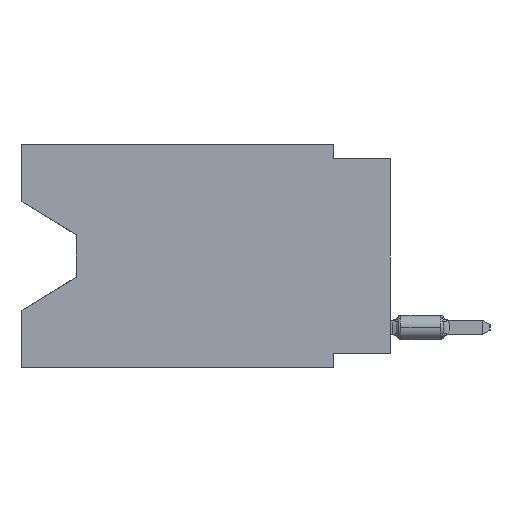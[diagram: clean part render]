
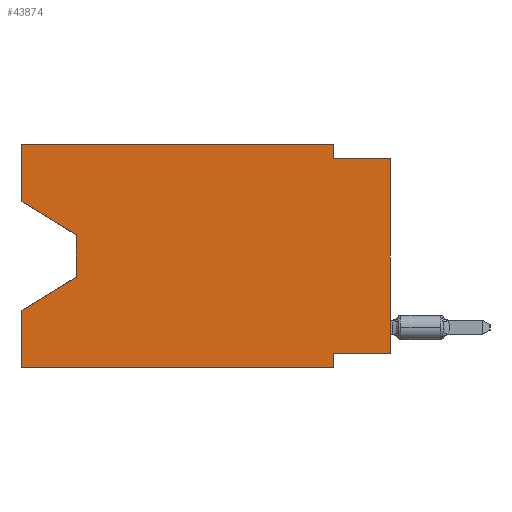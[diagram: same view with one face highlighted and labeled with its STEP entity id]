
A CAD part, left-side view. The second image highlights one B-rep face of the part: STEP entity #43874.
In plain terms, the highlighted planar face has unit normal (-1, 0, 0).
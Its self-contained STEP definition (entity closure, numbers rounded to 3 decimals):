
#273 = CARTESIAN_POINT ( 'NONE',  ( 0., 16.383, 0. ) ) ;
#1369 = LINE ( 'NONE', #19689, #4960 ) ;
#1424 = EDGE_LOOP ( 'NONE', ( #59179, #13717, #11758, #38852, #11616, #40115, #4180, #39235, #50964, #4521, #43627, #15643 ) ) ;
#2609 = CARTESIAN_POINT ( 'NONE',  ( 0., 16.383, -7.36 ) ) ;
#3058 = VERTEX_POINT ( 'NONE', #11367 ) ;
#3069 = CARTESIAN_POINT ( 'NONE',  ( 0., 16.383, 0. ) ) ;
#3442 = VECTOR ( 'NONE', #51423, 1000. ) ;
#4180 = ORIENTED_EDGE ( 'NONE', *, *, #4857, .F. ) ;
#4417 = DIRECTION ( 'NONE',  ( 0., 0., -1. ) ) ;
#4521 = ORIENTED_EDGE ( 'NONE', *, *, #47210, .F. ) ;
#4790 = EDGE_CURVE ( 'NONE', #7479, #24589, #44307, .T. ) ;
#4857 = EDGE_CURVE ( 'NONE', #54522, #42601, #21794, .T. ) ;
#4960 = VECTOR ( 'NONE', #56910, 1000. ) ;
#6357 = LINE ( 'NONE', #18962, #52579 ) ;
#6543 = EDGE_CURVE ( 'NONE', #7479, #56180, #6357, .T. ) ;
#6986 = PLANE ( 'NONE',  #28134 ) ;
#7234 = LINE ( 'NONE', #21036, #20885 ) ;
#7479 = VERTEX_POINT ( 'NONE', #23535 ) ;
#7560 = FACE_OUTER_BOUND ( 'NONE', #1424, .T. ) ;
#7615 = VECTOR ( 'NONE', #4417, 1000. ) ;
#8924 = CARTESIAN_POINT ( 'NONE',  ( 0., 2.54, 0. ) ) ;
#11367 = CARTESIAN_POINT ( 'NONE',  ( 0., 13.97, -4.013 ) ) ;
#11616 = ORIENTED_EDGE ( 'NONE', *, *, #6543, .T. ) ;
#11758 = ORIENTED_EDGE ( 'NONE', *, *, #39874, .T. ) ;
#12237 = EDGE_CURVE ( 'NONE', #42601, #56180, #15593, .T. ) ;
#13717 = ORIENTED_EDGE ( 'NONE', *, *, #21123, .T. ) ;
#13938 = EDGE_CURVE ( 'NONE', #53245, #50458, #7234, .T. ) ;
#15413 = DIRECTION ( 'NONE',  ( 0., -1., 0. ) ) ;
#15593 = LINE ( 'NONE', #33873, #49458 ) ;
#15643 = ORIENTED_EDGE ( 'NONE', *, *, #32635, .F. ) ;
#15814 = LINE ( 'NONE', #24511, #51469 ) ;
#18359 = VERTEX_POINT ( 'NONE', #46632 ) ;
#18466 = CARTESIAN_POINT ( 'NONE',  ( 0., 16.383, 0. ) ) ;
#18962 = CARTESIAN_POINT ( 'NONE',  ( 0., 16.383, -9.906 ) ) ;
#19046 = CARTESIAN_POINT ( 'NONE',  ( 0., 2.54, -9.906 ) ) ;
#19356 = VERTEX_POINT ( 'NONE', #38285 ) ;
#19689 = CARTESIAN_POINT ( 'NONE',  ( 0., 16.383, -2.546 ) ) ;
#20840 = VECTOR ( 'NONE', #53907, 1000. ) ;
#20885 = VECTOR ( 'NONE', #53433, 1000. ) ;
#21036 = CARTESIAN_POINT ( 'NONE',  ( 0., 0., -0.635 ) ) ;
#21123 = EDGE_CURVE ( 'NONE', #3058, #40412, #29351, .T. ) ;
#21794 = LINE ( 'NONE', #40097, #20840 ) ;
#23535 = CARTESIAN_POINT ( 'NONE',  ( 0., 16.383, -9.906 ) ) ;
#23709 = VECTOR ( 'NONE', #49681, 1000. ) ;
#23934 = EDGE_CURVE ( 'NONE', #42138, #19356, #33990, .T. ) ;
#24511 = CARTESIAN_POINT ( 'NONE',  ( 0., 13.97, -5.893 ) ) ;
#24589 = VERTEX_POINT ( 'NONE', #2609 ) ;
#25166 = VECTOR ( 'NONE', #51147, 1000. ) ;
#25289 = DIRECTION ( 'NONE',  ( 1., 0., 0. ) ) ;
#27185 = VECTOR ( 'NONE', #48545, 1000. ) ;
#27235 = CARTESIAN_POINT ( 'NONE',  ( 0., 2.54, -9.271 ) ) ;
#27745 = CARTESIAN_POINT ( 'NONE',  ( 0., 0., 0. ) ) ;
#28134 = AXIS2_PLACEMENT_3D ( 'NONE', #3069, #25289, #43570 ) ;
#28212 = CARTESIAN_POINT ( 'NONE',  ( 0., 2.54, -0.635 ) ) ;
#29351 = LINE ( 'NONE', #53070, #27185 ) ;
#30650 = EDGE_CURVE ( 'NONE', #54522, #50458, #36765, .T. ) ;
#32139 = CARTESIAN_POINT ( 'NONE',  ( 0., 0., -9.271 ) ) ;
#32635 = EDGE_CURVE ( 'NONE', #18359, #42138, #37034, .T. ) ;
#33873 = CARTESIAN_POINT ( 'NONE',  ( 0., 2.54, -9.906 ) ) ;
#33990 = LINE ( 'NONE', #56517, #46785 ) ;
#34685 = CARTESIAN_POINT ( 'NONE',  ( 0., 0., -0.635 ) ) ;
#36765 = LINE ( 'NONE', #27745, #25166 ) ;
#37034 = LINE ( 'NONE', #18466, #3442 ) ;
#38285 = CARTESIAN_POINT ( 'NONE',  ( 0., 2.54, 0. ) ) ;
#38852 = ORIENTED_EDGE ( 'NONE', *, *, #4790, .F. ) ;
#39235 = ORIENTED_EDGE ( 'NONE', *, *, #30650, .T. ) ;
#39874 = EDGE_CURVE ( 'NONE', #40412, #24589, #15814, .T. ) ;
#40097 = CARTESIAN_POINT ( 'NONE',  ( 0., 0., -9.271 ) ) ;
#40115 = ORIENTED_EDGE ( 'NONE', *, *, #12237, .F. ) ;
#40412 = VERTEX_POINT ( 'NONE', #57400 ) ;
#42138 = VERTEX_POINT ( 'NONE', #273 ) ;
#42601 = VERTEX_POINT ( 'NONE', #27235 ) ;
#43097 = DIRECTION ( 'NONE',  ( 0., 0.855, -0.519 ) ) ;
#43570 = DIRECTION ( 'NONE',  ( 0., 0., -1. ) ) ;
#43627 = ORIENTED_EDGE ( 'NONE', *, *, #23934, .F. ) ;
#43874 = ADVANCED_FACE ( 'NONE', ( #7560 ), #6986, .F. ) ;
#44307 = LINE ( 'NONE', #58724, #23709 ) ;
#46632 = CARTESIAN_POINT ( 'NONE',  ( 0., 16.383, -2.546 ) ) ;
#46785 = VECTOR ( 'NONE', #15413, 1000. ) ;
#47210 = EDGE_CURVE ( 'NONE', #19356, #53245, #54545, .T. ) ;
#48545 = DIRECTION ( 'NONE',  ( 0., 0., -1. ) ) ;
#49244 = EDGE_CURVE ( 'NONE', #18359, #3058, #1369, .T. ) ;
#49458 = VECTOR ( 'NONE', #52184, 1000. ) ;
#49681 = DIRECTION ( 'NONE',  ( 0., 0., 1. ) ) ;
#50458 = VERTEX_POINT ( 'NONE', #34685 ) ;
#50964 = ORIENTED_EDGE ( 'NONE', *, *, #13938, .F. ) ;
#51147 = DIRECTION ( 'NONE',  ( 0., 0., 1. ) ) ;
#51423 = DIRECTION ( 'NONE',  ( 0., 0., 1. ) ) ;
#51469 = VECTOR ( 'NONE', #43097, 1000. ) ;
#52184 = DIRECTION ( 'NONE',  ( 0., 0., -1. ) ) ;
#52579 = VECTOR ( 'NONE', #55900, 1000. ) ;
#53070 = CARTESIAN_POINT ( 'NONE',  ( 0., 13.97, -4.013 ) ) ;
#53245 = VERTEX_POINT ( 'NONE', #28212 ) ;
#53433 = DIRECTION ( 'NONE',  ( 0., -1., 0. ) ) ;
#53907 = DIRECTION ( 'NONE',  ( 0., 1., 0. ) ) ;
#54522 = VERTEX_POINT ( 'NONE', #32139 ) ;
#54545 = LINE ( 'NONE', #8924, #7615 ) ;
#55900 = DIRECTION ( 'NONE',  ( 0., -1., 0. ) ) ;
#56180 = VERTEX_POINT ( 'NONE', #19046 ) ;
#56517 = CARTESIAN_POINT ( 'NONE',  ( 0., 16.383, 0. ) ) ;
#56910 = DIRECTION ( 'NONE',  ( 0., -0.855, -0.519 ) ) ;
#57400 = CARTESIAN_POINT ( 'NONE',  ( 0., 13.97, -5.893 ) ) ;
#58724 = CARTESIAN_POINT ( 'NONE',  ( 0., 16.383, 0. ) ) ;
#59179 = ORIENTED_EDGE ( 'NONE', *, *, #49244, .T. ) ;
